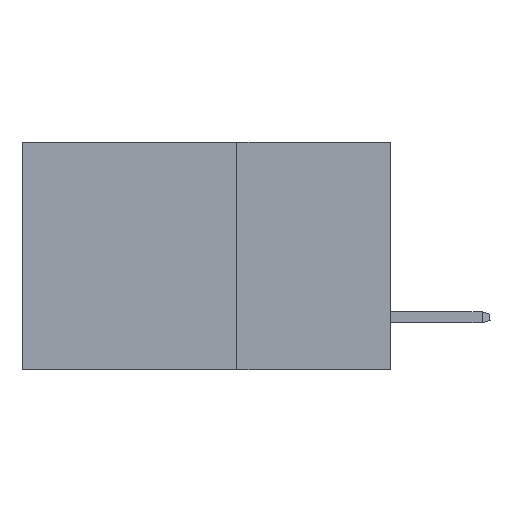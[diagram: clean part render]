
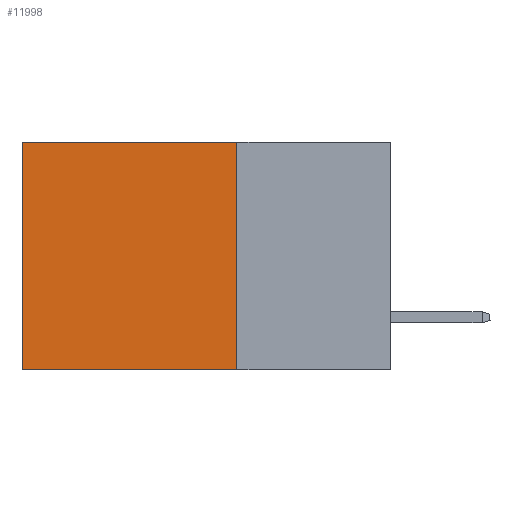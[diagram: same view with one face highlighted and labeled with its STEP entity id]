
A CAD part, left-side view. The second image highlights one B-rep face of the part: STEP entity #11998.
In plain terms, the highlighted planar face has unit normal (-1, 0, 0).
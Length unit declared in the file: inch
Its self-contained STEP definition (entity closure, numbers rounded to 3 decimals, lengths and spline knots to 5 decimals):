
#471 = EDGE_CURVE ( 'NONE', #13597, #16823, #5032, .T. ) ;
#879 = DIRECTION ( 'NONE',  ( 0., 0., -1. ) ) ;
#960 = CARTESIAN_POINT ( 'NONE',  ( 0.2875, 0.6, 0. ) ) ;
#1320 = ORIENTED_EDGE ( 'NONE', *, *, #471, .T. ) ;
#2293 = LINE ( 'NONE', #9056, #5053 ) ;
#2560 = LINE ( 'NONE', #5253, #9767 ) ;
#3181 = ORIENTED_EDGE ( 'NONE', *, *, #6922, .T. ) ;
#3993 = CARTESIAN_POINT ( 'NONE',  ( 0.2875, 0.25, 0. ) ) ;
#4466 = FACE_OUTER_BOUND ( 'NONE', #16703, .T. ) ;
#4565 = DIRECTION ( 'NONE',  ( 0., 0., -1. ) ) ;
#5032 = LINE ( 'NONE', #960, #11216 ) ;
#5053 = VECTOR ( 'NONE', #17479, 39.37008 ) ;
#5253 = CARTESIAN_POINT ( 'NONE',  ( 0.2875, 0.25, -0.37 ) ) ;
#5914 = DIRECTION ( 'NONE',  ( 1., 0., 0. ) ) ;
#6695 = DIRECTION ( 'NONE',  ( 0., 0., -1. ) ) ;
#6884 = LINE ( 'NONE', #8148, #13149 ) ;
#6922 = EDGE_CURVE ( 'NONE', #13074, #13597, #2293, .T. ) ;
#6990 = EDGE_CURVE ( 'NONE', #13074, #13825, #6884, .T. ) ;
#7932 = AXIS2_PLACEMENT_3D ( 'NONE', #8642, #5914, #4565 ) ;
#8148 = CARTESIAN_POINT ( 'NONE',  ( 0.2875, 0.25, 0. ) ) ;
#8642 = CARTESIAN_POINT ( 'NONE',  ( 0.2875, 0.25, 0. ) ) ;
#9056 = CARTESIAN_POINT ( 'NONE',  ( 0.2875, 0.25, 0. ) ) ;
#9767 = VECTOR ( 'NONE', #16567, 39.37008 ) ;
#9906 = CARTESIAN_POINT ( 'NONE',  ( 0.2875, 0.6, -0.37 ) ) ;
#9988 = PLANE ( 'NONE',  #7932 ) ;
#11216 = VECTOR ( 'NONE', #879, 39.37008 ) ;
#11998 = ADVANCED_FACE ( 'NONE', ( #4466 ), #9988, .F. ) ;
#12976 = ORIENTED_EDGE ( 'NONE', *, *, #17751, .F. ) ;
#13074 = VERTEX_POINT ( 'NONE', #3993 ) ;
#13149 = VECTOR ( 'NONE', #6695, 39.37008 ) ;
#13538 = CARTESIAN_POINT ( 'NONE',  ( 0.2875, 0.6, 0. ) ) ;
#13597 = VERTEX_POINT ( 'NONE', #13538 ) ;
#13825 = VERTEX_POINT ( 'NONE', #15617 ) ;
#15617 = CARTESIAN_POINT ( 'NONE',  ( 0.2875, 0.25, -0.37 ) ) ;
#16464 = ORIENTED_EDGE ( 'NONE', *, *, #6990, .F. ) ;
#16567 = DIRECTION ( 'NONE',  ( 0., 1., 0. ) ) ;
#16703 = EDGE_LOOP ( 'NONE', ( #1320, #12976, #16464, #3181 ) ) ;
#16823 = VERTEX_POINT ( 'NONE', #9906 ) ;
#17479 = DIRECTION ( 'NONE',  ( 0., 1., 0. ) ) ;
#17751 = EDGE_CURVE ( 'NONE', #13825, #16823, #2560, .T. ) ;
